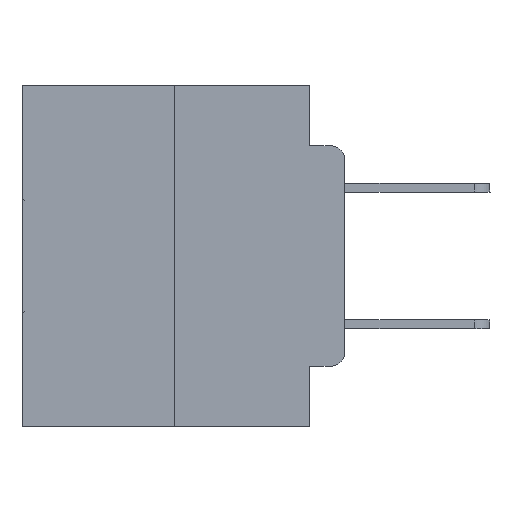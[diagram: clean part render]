
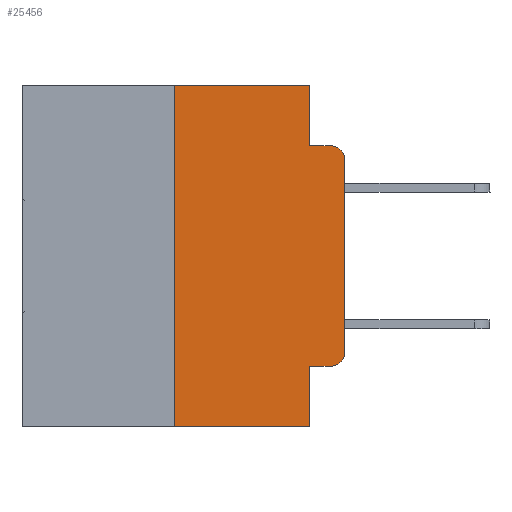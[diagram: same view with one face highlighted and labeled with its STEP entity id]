
A CAD part, left-side view. The second image highlights one B-rep face of the part: STEP entity #25456.
In plain terms, the highlighted planar face has unit normal (-1, 0, 0).
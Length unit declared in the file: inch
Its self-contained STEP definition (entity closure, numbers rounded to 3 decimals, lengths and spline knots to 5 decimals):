
#393 = CARTESIAN_POINT ( 'NONE',  ( 0., 0.02, -0.0885 ) ) ;
#687 = CARTESIAN_POINT ( 'NONE',  ( 0., 0.051, -0.4115 ) ) ;
#841 = VECTOR ( 'NONE', #25269, 39.37008 ) ;
#896 = DIRECTION ( 'NONE',  ( 0., -1., 0. ) ) ;
#1365 = VECTOR ( 'NONE', #2108, 39.37008 ) ;
#1367 = VECTOR ( 'NONE', #12875, 39.37008 ) ;
#1475 = ORIENTED_EDGE ( 'NONE', *, *, #21592, .F. ) ;
#1706 = PLANE ( 'NONE',  #12562 ) ;
#2108 = DIRECTION ( 'NONE',  ( 0., 0., 1. ) ) ;
#2138 = CARTESIAN_POINT ( 'NONE',  ( 0., 0.051, -0.0885 ) ) ;
#3492 = VECTOR ( 'NONE', #896, 39.37008 ) ;
#3642 = CARTESIAN_POINT ( 'NONE',  ( 0., 0.25, 0. ) ) ;
#3848 = AXIS2_PLACEMENT_3D ( 'NONE', #6987, #5560, #14829 ) ;
#4255 = VERTEX_POINT ( 'NONE', #393 ) ;
#4291 = CIRCLE ( 'NONE', #18849, 0.02 ) ;
#4424 = VERTEX_POINT ( 'NONE', #9969 ) ;
#4651 = ORIENTED_EDGE ( 'NONE', *, *, #9256, .T. ) ;
#5331 = CARTESIAN_POINT ( 'NONE',  ( 0., 0.051, -0.4115 ) ) ;
#5560 = DIRECTION ( 'NONE',  ( -1., 0., 0. ) ) ;
#5737 = CARTESIAN_POINT ( 'NONE',  ( 0., 0.051, 0. ) ) ;
#6964 = CARTESIAN_POINT ( 'NONE',  ( 0., 0.25, -0.5 ) ) ;
#6987 = CARTESIAN_POINT ( 'NONE',  ( 0., 0.02, -0.1085 ) ) ;
#7114 = CARTESIAN_POINT ( 'NONE',  ( 0., 0.02, -0.3915 ) ) ;
#7410 = DIRECTION ( 'NONE',  ( 0., -1., 0. ) ) ;
#7449 = LINE ( 'NONE', #5331, #24707 ) ;
#7593 = VECTOR ( 'NONE', #7410, 39.37008 ) ;
#8580 = CARTESIAN_POINT ( 'NONE',  ( 0., 0.051, 0. ) ) ;
#8681 = VECTOR ( 'NONE', #30082, 39.37008 ) ;
#8922 = ORIENTED_EDGE ( 'NONE', *, *, #10717, .F. ) ;
#8927 = LINE ( 'NONE', #22776, #8681 ) ;
#9256 = EDGE_CURVE ( 'NONE', #27899, #4424, #7449, .T. ) ;
#9265 = LINE ( 'NONE', #29966, #841 ) ;
#9488 = EDGE_CURVE ( 'NONE', #4424, #16359, #4291, .T. ) ;
#9705 = CARTESIAN_POINT ( 'NONE',  ( 0., 0.473, 0. ) ) ;
#9858 = EDGE_CURVE ( 'NONE', #22353, #10459, #29483, .T. ) ;
#9969 = CARTESIAN_POINT ( 'NONE',  ( 0., 0.02, -0.4115 ) ) ;
#10290 = ORIENTED_EDGE ( 'NONE', *, *, #26050, .T. ) ;
#10459 = VERTEX_POINT ( 'NONE', #2138 ) ;
#10717 = EDGE_CURVE ( 'NONE', #21526, #20944, #20395, .T. ) ;
#10725 = CARTESIAN_POINT ( 'NONE',  ( 0., 0.051, -0.5 ) ) ;
#10931 = EDGE_CURVE ( 'NONE', #16359, #20288, #17318, .T. ) ;
#11088 = VECTOR ( 'NONE', #13373, 39.37008 ) ;
#11343 = EDGE_CURVE ( 'NONE', #21526, #16168, #8927, .T. ) ;
#12167 = CARTESIAN_POINT ( 'NONE',  ( 0., 0., -0.3915 ) ) ;
#12562 = AXIS2_PLACEMENT_3D ( 'NONE', #17991, #15988, #22410 ) ;
#12853 = ORIENTED_EDGE ( 'NONE', *, *, #22792, .F. ) ;
#12875 = DIRECTION ( 'NONE',  ( 0., 0., -1. ) ) ;
#13032 = ORIENTED_EDGE ( 'NONE', *, *, #10931, .T. ) ;
#13373 = DIRECTION ( 'NONE',  ( 0., 0., 1. ) ) ;
#14191 = EDGE_LOOP ( 'NONE', ( #13032, #10290, #26129, #24790, #1475, #8922, #22450, #12853, #4651, #19124 ) ) ;
#14440 = LINE ( 'NONE', #17041, #3492 ) ;
#14829 = DIRECTION ( 'NONE',  ( 0., 0., -1. ) ) ;
#15988 = DIRECTION ( 'NONE',  ( 1., 0., 0. ) ) ;
#16168 = VERTEX_POINT ( 'NONE', #10725 ) ;
#16359 = VERTEX_POINT ( 'NONE', #12167 ) ;
#16385 = DIRECTION ( 'NONE',  ( 0., 0., -1. ) ) ;
#16436 = EDGE_CURVE ( 'NONE', #10459, #4255, #14440, .T. ) ;
#16951 = CIRCLE ( 'NONE', #3848, 0.02 ) ;
#17041 = CARTESIAN_POINT ( 'NONE',  ( 0., 0.051, -0.0885 ) ) ;
#17318 = LINE ( 'NONE', #29970, #1365 ) ;
#17835 = FACE_OUTER_BOUND ( 'NONE', #14191, .T. ) ;
#17991 = CARTESIAN_POINT ( 'NONE',  ( 0., 0.473, 0. ) ) ;
#18813 = LINE ( 'NONE', #9705, #7593 ) ;
#18849 = AXIS2_PLACEMENT_3D ( 'NONE', #7114, #27546, #16385 ) ;
#19124 = ORIENTED_EDGE ( 'NONE', *, *, #9488, .T. ) ;
#20288 = VERTEX_POINT ( 'NONE', #27518 ) ;
#20395 = LINE ( 'NONE', #3642, #11088 ) ;
#20944 = VERTEX_POINT ( 'NONE', #28513 ) ;
#21526 = VERTEX_POINT ( 'NONE', #6964 ) ;
#21592 = EDGE_CURVE ( 'NONE', #20944, #22353, #18813, .T. ) ;
#22353 = VERTEX_POINT ( 'NONE', #8580 ) ;
#22410 = DIRECTION ( 'NONE',  ( 0., 0., -1. ) ) ;
#22450 = ORIENTED_EDGE ( 'NONE', *, *, #11343, .T. ) ;
#22776 = CARTESIAN_POINT ( 'NONE',  ( 0., 0.473, -0.5 ) ) ;
#22792 = EDGE_CURVE ( 'NONE', #27899, #16168, #9265, .T. ) ;
#24707 = VECTOR ( 'NONE', #26484, 39.37008 ) ;
#24790 = ORIENTED_EDGE ( 'NONE', *, *, #9858, .F. ) ;
#25269 = DIRECTION ( 'NONE',  ( 0., 0., -1. ) ) ;
#25456 = ADVANCED_FACE ( 'NONE', ( #17835 ), #1706, .F. ) ;
#26050 = EDGE_CURVE ( 'NONE', #20288, #4255, #16951, .T. ) ;
#26129 = ORIENTED_EDGE ( 'NONE', *, *, #16436, .F. ) ;
#26484 = DIRECTION ( 'NONE',  ( 0., -1., 0. ) ) ;
#27518 = CARTESIAN_POINT ( 'NONE',  ( 0., 0., -0.1085 ) ) ;
#27546 = DIRECTION ( 'NONE',  ( -1., 0., 0. ) ) ;
#27899 = VERTEX_POINT ( 'NONE', #687 ) ;
#28513 = CARTESIAN_POINT ( 'NONE',  ( 0., 0.25, 0. ) ) ;
#29483 = LINE ( 'NONE', #5737, #1367 ) ;
#29966 = CARTESIAN_POINT ( 'NONE',  ( 0., 0.051, 0. ) ) ;
#29970 = CARTESIAN_POINT ( 'NONE',  ( 0., 0., 0. ) ) ;
#30082 = DIRECTION ( 'NONE',  ( 0., -1., 0. ) ) ;
